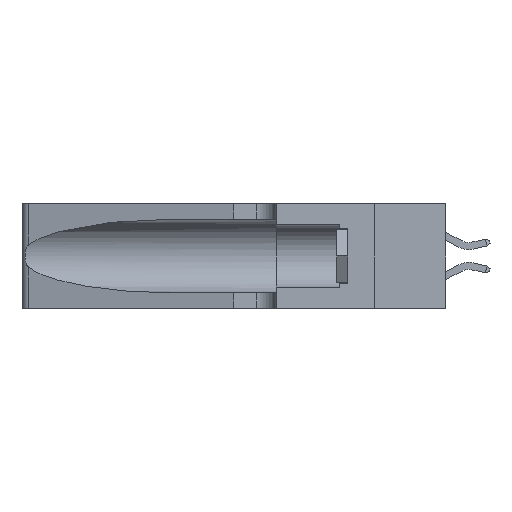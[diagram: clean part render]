
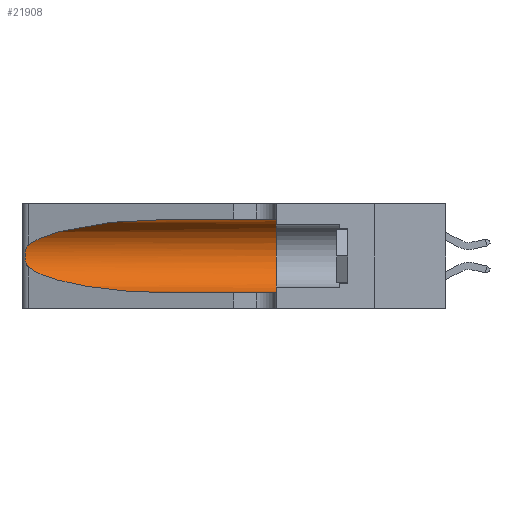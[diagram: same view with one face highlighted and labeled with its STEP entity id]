
A CAD part, left-side view. The second image highlights one B-rep face of the part: STEP entity #21908.
In plain terms, the highlighted cylindrical face has radius 3.308 mm (diameter 6.617 mm), a partial arc.
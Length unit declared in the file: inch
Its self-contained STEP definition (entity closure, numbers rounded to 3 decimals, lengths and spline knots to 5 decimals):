
#898 = CARTESIAN_POINT ( 'NONE',  ( 0.25555, 1.22993, 0.14849 ) ) ;
#1094 = EDGE_CURVE ( 'NONE', #13077, #8137, #27029, .T. ) ;
#1105 = CARTESIAN_POINT ( 'NONE',  ( 0.1305, 0.35, 0.05475 ) ) ;
#1148 = EDGE_CURVE ( 'NONE', #1327, #34812, #32752, .T. ) ;
#1327 = VERTEX_POINT ( 'NONE', #35533 ) ;
#2706 = EDGE_CURVE ( 'NONE', #1327, #13077, #30364, .T. ) ;
#2948 = CARTESIAN_POINT ( 'NONE',  ( 0.1305, 0.72297, 0.31525 ) ) ;
#3671 = DIRECTION ( 'NONE',  ( 0., -1., 0. ) ) ;
#4547 = AXIS2_PLACEMENT_3D ( 'NONE', #37703, #34258, #40679 ) ;
#4697 = CARTESIAN_POINT ( 'NONE',  ( 0.1305, 1.61858, 0.05475 ) ) ;
#4832 = CARTESIAN_POINT ( 'NONE',  ( 0.25555, 1.22994, 0.2215 ) ) ;
#5707 = VERTEX_POINT ( 'NONE', #20705 ) ;
#6839 = CARTESIAN_POINT ( 'NONE',  ( 0.1305, 0.35, 0.31525 ) ) ;
#7163 = ORIENTED_EDGE ( 'NONE', *, *, #30898, .T. ) ;
#7284 = CARTESIAN_POINT ( 'NONE',  ( 0.25487, 1.22718, 0.22369 ) ) ;
#7314 = CARTESIAN_POINT ( 'NONE',  ( 0.2373, 1.15595, 0.08982 ) ) ;
#7443 = CARTESIAN_POINT ( 'NONE',  ( 0.25487, 1.22718, 0.14631 ) ) ;
#8137 = VERTEX_POINT ( 'NONE', #1105 ) ;
#8152 = AXIS2_PLACEMENT_3D ( 'NONE', #22696, #3671, #26191 ) ;
#8176 = ORIENTED_EDGE ( 'NONE', *, *, #31482, .T. ) ;
#8547 = CARTESIAN_POINT ( 'NONE',  ( 0.25487, 1.22718, 0.14631 ) ) ;
#9279 = CARTESIAN_POINT ( 'NONE',  ( 0.25487, 1.22718, 0.22369 ) ) ;
#10518 = CARTESIAN_POINT ( 'NONE',  ( 0.1305, 0.72297, 0.05475 ) ) ;
#11706 = ORIENTED_EDGE ( 'NONE', *, *, #21193, .T. ) ;
#12138 = LINE ( 'NONE', #4697, #40567 ) ;
#12604 = CYLINDRICAL_SURFACE ( 'NONE', #8152, 0.13025 ) ;
#13077 = VERTEX_POINT ( 'NONE', #6839 ) ;
#13573 = B_SPLINE_CURVE_WITH_KNOTS ( 'NONE', 3,
 ( #7284, #4832, #27095, #30304, #36288, #17433, #20570, #21663, #31609, #16371, #28837, #16230, #898, #29129 ),
 .UNSPECIFIED., .F., .F.,
 ( 4, 2, 2, 2, 2, 2, 4 ),
 ( 0., 0.00027, 0.00053, 0.00107, 0.0016, 0.00187, 0.00214 ),
 .UNSPECIFIED. ) ;
#13954 = ORIENTED_EDGE ( 'NONE', *, *, #1094, .F. ) ;
#16230 = CARTESIAN_POINT ( 'NONE',  ( 0.25639, 1.23186, 0.15144 ) ) ;
#16371 = CARTESIAN_POINT ( 'NONE',  ( 0.25856, 1.23593, 0.16098 ) ) ;
#17433 = CARTESIAN_POINT ( 'NONE',  ( 0.26018, 1.23835, 0.19895 ) ) ;
#17601 = DIRECTION ( 'NONE',  ( 0., -1., 0. ) ) ;
#19045 = FACE_OUTER_BOUND ( 'NONE', #24139, .T. ) ;
#19172 = DIRECTION ( 'NONE',  ( 0., -1., 0. ) ) ;
#20407 = ORIENTED_EDGE ( 'NONE', *, *, #1148, .T. ) ;
#20570 = CARTESIAN_POINT ( 'NONE',  ( 0.26075, 1.23896, 0.19203 ) ) ;
#20705 = CARTESIAN_POINT ( 'NONE',  ( 0.1305, 0.72297, 0.05475 ) ) ;
#21193 = EDGE_CURVE ( 'NONE', #34812, #39488, #13573, .T. ) ;
#21663 = CARTESIAN_POINT ( 'NONE',  ( 0.26075, 1.23896, 0.178 ) ) ;
#21844 = VECTOR ( 'NONE', #19172, 39.37008 ) ;
#21908 = ADVANCED_FACE ( 'NONE', ( #19045 ), #12604, .F. ) ;
#22081 = CARTESIAN_POINT ( 'NONE',  ( 0.2373, 1.15595, 0.28018 ) ) ;
#22696 = CARTESIAN_POINT ( 'NONE',  ( 0.1305, 1.61858, 0.185 ) ) ;
#24139 = EDGE_LOOP ( 'NONE', ( #20407, #11706, #7163, #8176, #13954, #38283 ) ) ;
#26191 = DIRECTION ( 'NONE',  ( 0., 0., -1. ) ) ;
#26527 =( BOUNDED_CURVE ( )  B_SPLINE_CURVE ( 3, ( #7443, #7314, #29647, #10518 ),
 .UNSPECIFIED., .F., .T. ) 
 B_SPLINE_CURVE_WITH_KNOTS ( ( 4, 4 ),
 ( 3.44316, 4.71239 ),
 .UNSPECIFIED. ) 
 CURVE ( )  GEOMETRIC_REPRESENTATION_ITEM ( )  RATIONAL_B_SPLINE_CURVE ( ( 1., 0.87, 0.87, 1. ) ) 
 REPRESENTATION_ITEM ( '' )  );
#27029 = CIRCLE ( 'NONE', #4547, 0.13025 ) ;
#27095 = CARTESIAN_POINT ( 'NONE',  ( 0.25639, 1.23184, 0.21858 ) ) ;
#27356 = CARTESIAN_POINT ( 'NONE',  ( 0.25487, 1.22718, 0.22369 ) ) ;
#28837 = CARTESIAN_POINT ( 'NONE',  ( 0.25789, 1.23486, 0.15765 ) ) ;
#29129 = CARTESIAN_POINT ( 'NONE',  ( 0.25487, 1.22718, 0.14631 ) ) ;
#29249 = CARTESIAN_POINT ( 'NONE',  ( 0.1305, 1.61858, 0.31525 ) ) ;
#29647 = CARTESIAN_POINT ( 'NONE',  ( 0.18966, 0.96281, 0.05475 ) ) ;
#30304 = CARTESIAN_POINT ( 'NONE',  ( 0.25787, 1.23484, 0.2124 ) ) ;
#30364 = LINE ( 'NONE', #29249, #21844 ) ;
#30898 = EDGE_CURVE ( 'NONE', #39488, #5707, #26527, .T. ) ;
#31482 = EDGE_CURVE ( 'NONE', #5707, #8137, #12138, .T. ) ;
#31609 = CARTESIAN_POINT ( 'NONE',  ( 0.26017, 1.23833, 0.17102 ) ) ;
#32752 =( BOUNDED_CURVE ( )  B_SPLINE_CURVE ( 3, ( #2948, #37835, #22081, #9279 ),
 .UNSPECIFIED., .F., .F. ) 
 B_SPLINE_CURVE_WITH_KNOTS ( ( 4, 4 ),
 ( 1.5708, 2.84003 ),
 .UNSPECIFIED. ) 
 CURVE ( )  GEOMETRIC_REPRESENTATION_ITEM ( )  RATIONAL_B_SPLINE_CURVE ( ( 1., 0.87, 0.87, 1. ) ) 
 REPRESENTATION_ITEM ( '' )  );
#34258 = DIRECTION ( 'NONE',  ( 0., 1., 0. ) ) ;
#34812 = VERTEX_POINT ( 'NONE', #27356 ) ;
#35533 = CARTESIAN_POINT ( 'NONE',  ( 0.1305, 0.72297, 0.31525 ) ) ;
#36288 = CARTESIAN_POINT ( 'NONE',  ( 0.25854, 1.2359, 0.20912 ) ) ;
#37703 = CARTESIAN_POINT ( 'NONE',  ( 0.1305, 0.35, 0.185 ) ) ;
#37835 = CARTESIAN_POINT ( 'NONE',  ( 0.18966, 0.96281, 0.31525 ) ) ;
#38283 = ORIENTED_EDGE ( 'NONE', *, *, #2706, .F. ) ;
#39488 = VERTEX_POINT ( 'NONE', #8547 ) ;
#40567 = VECTOR ( 'NONE', #17601, 39.37008 ) ;
#40679 = DIRECTION ( 'NONE',  ( 0., 0., 1. ) ) ;
